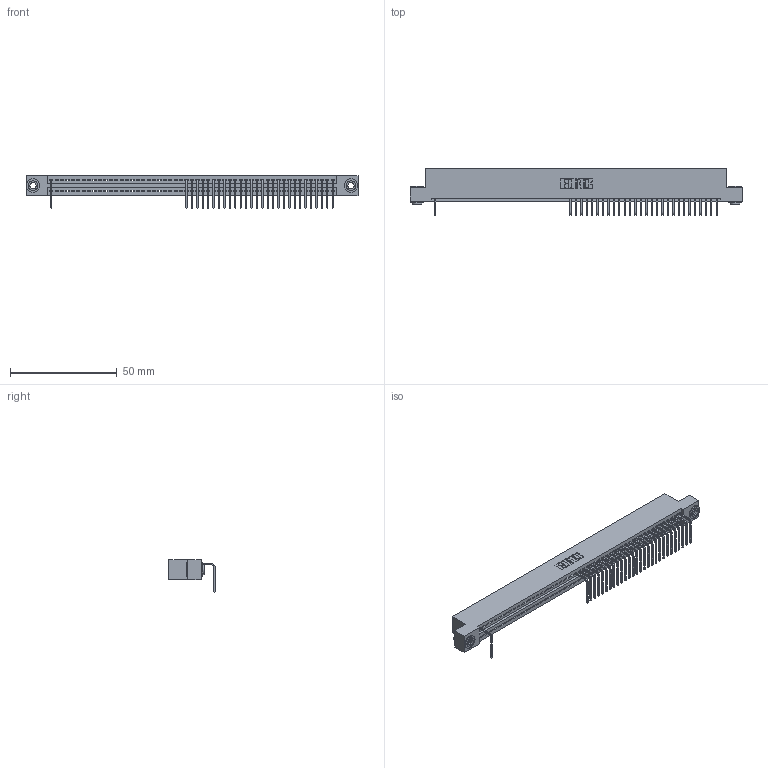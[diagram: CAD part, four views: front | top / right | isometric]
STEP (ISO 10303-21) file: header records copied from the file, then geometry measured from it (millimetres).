
FILE_DESCRIPTION (( 'STEP AP203' ), '1' );
FILE_NAME ('345-053-558-103.STEP', '2018-09-23T19:02:01', ( '' ), ( '' ), 'SwSTEP 2.0', 'SolidWorks 2016', '' );
FILE_SCHEMA (( 'CONFIG_CONTROL_DESIGN' ));
Length unit declared in the file: inch
Products named in the file (4): 345-053-558-103; 345 Part_Flush Mounting Lugs - 0.156 Dia-TH; 345-292-001_558 Tail - 2; 345-250-002_345-250-002-102
Assembly tree (32 placements, depth 2):
  345-053-558-103
    345 Part_Flush Mounting Lugs - 0.156 Dia-TH
    345-292-001_558 Tail - 2  x29
    345-250-002_345-250-002-102  x2
Bounding box: 155.83 x 21.83 x 15.37 mm (x, y, z)
Volume: 14732.1 mm3; surface area: 19049.9 mm2
Topology: 32 solids, 32 shells, 2288 faces, 6991 edges, 4618 vertices
Faces by surface type: plane 1644, cylinder 636, cone 8
Entity records: 38374 total; most frequent: ORIENTED_EDGE 6738, CARTESIAN_POINT 6734, DIRECTION 5869, EDGE_CURVE 3369, VECTOR 3001, LINE 3001, VERTEX_POINT 2242, AXIS2_PLACEMENT_3D 1434
